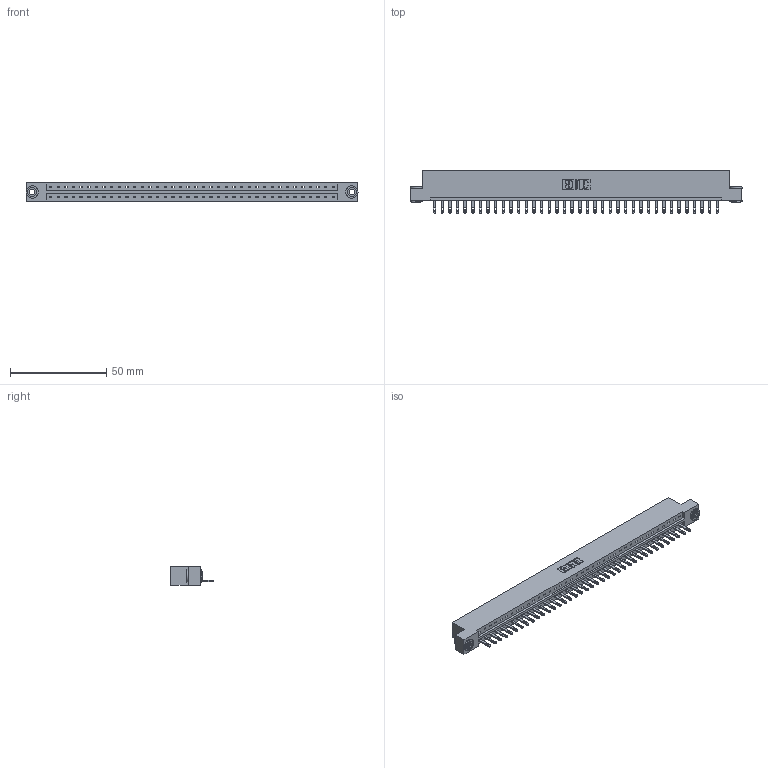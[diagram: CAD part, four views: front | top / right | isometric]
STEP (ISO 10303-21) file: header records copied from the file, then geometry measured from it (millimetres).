
FILE_DESCRIPTION (( 'STEP AP203' ), '1' );
FILE_NAME ('833-038-500-103.STEP', '2020-06-03T06:01:21', ( '' ), ( '' ), 'SwSTEP 2.0', 'SolidWorks 2020', '' );
FILE_SCHEMA (( 'CONFIG_CONTROL_DESIGN' ));
Length unit declared in the file: inch
Products named in the file (4): 833 Part_Flush - .156 Dia - TH; 833-038-500-103; 345-250-002_345-250-002-102; 345-292-001_345-293-100
Assembly tree (41 placements, depth 2):
  833-038-500-103
    833 Part_Flush - .156 Dia - TH
    345-292-001_345-293-100  x38
    345-250-002_345-250-002-102  x2
Bounding box: 172.11 x 21.85 x 9.4 mm (x, y, z)
Volume: 17327.7 mm3; surface area: 19042 mm2
Topology: 41 solids, 41 shells, 2204 faces, 6771 edges, 4510 vertices
Faces by surface type: plane 1448, cylinder 748, cone 8
Entity records: 24328 total; most frequent: CARTESIAN_POINT 4175, ORIENTED_EDGE 4142, DIRECTION 3565, EDGE_CURVE 2071, VECTOR 1915, LINE 1915, VERTEX_POINT 1378, AXIS2_PLACEMENT_3D 825
